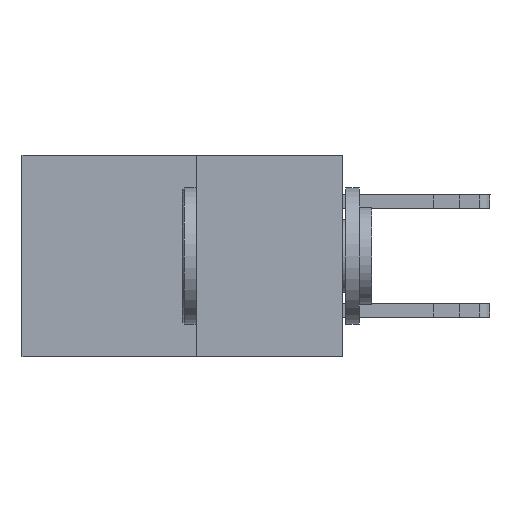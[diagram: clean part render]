
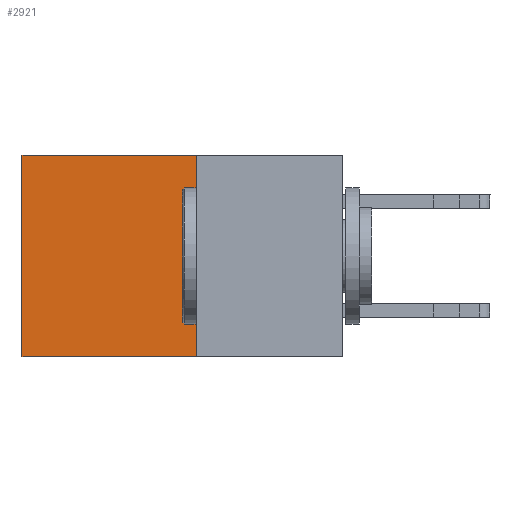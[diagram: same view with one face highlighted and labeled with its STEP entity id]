
A CAD part, left-side view. The second image highlights one B-rep face of the part: STEP entity #2921.
In plain terms, the highlighted planar face has unit normal (-1, 0, 0).
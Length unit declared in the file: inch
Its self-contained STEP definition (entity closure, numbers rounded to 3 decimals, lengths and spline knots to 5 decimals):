
#96 = LINE ( 'NONE', #9921, #3054 ) ;
#958 = VECTOR ( 'NONE', #9439, 39.37008 ) ;
#1492 = DIRECTION ( 'NONE',  ( 0., 0., -1. ) ) ;
#1629 = CARTESIAN_POINT ( 'NONE',  ( 0.277, 0.27, -0.37 ) ) ;
#1982 = DIRECTION ( 'NONE',  ( 0., 0., -1. ) ) ;
#2193 = VERTEX_POINT ( 'NONE', #3364 ) ;
#2755 = VECTOR ( 'NONE', #5610, 39.37008 ) ;
#2921 = ADVANCED_FACE ( 'NONE', ( #11876 ), #14265, .F. ) ;
#3054 = VECTOR ( 'NONE', #1492, 39.37008 ) ;
#3336 = AXIS2_PLACEMENT_3D ( 'NONE', #6869, #14428, #7793 ) ;
#3364 = CARTESIAN_POINT ( 'NONE',  ( 0.277, 0.27, 0. ) ) ;
#4204 = ORIENTED_EDGE ( 'NONE', *, *, #13382, .T. ) ;
#4409 = VECTOR ( 'NONE', #1982, 39.37008 ) ;
#5209 = ORIENTED_EDGE ( 'NONE', *, *, #8585, .F. ) ;
#5610 = DIRECTION ( 'NONE',  ( 0., 1., 0. ) ) ;
#5645 = EDGE_CURVE ( 'NONE', #5677, #10292, #15283, .T. ) ;
#5647 = CARTESIAN_POINT ( 'NONE',  ( 0.277, 0.59, -0.37 ) ) ;
#5677 = VERTEX_POINT ( 'NONE', #1629 ) ;
#6869 = CARTESIAN_POINT ( 'NONE',  ( 0.277, 0.27, -0.37 ) ) ;
#7793 = DIRECTION ( 'NONE',  ( 0., 0., -1. ) ) ;
#7897 = EDGE_LOOP ( 'NONE', ( #11575, #10295, #5209, #4204 ) ) ;
#8185 = CARTESIAN_POINT ( 'NONE',  ( 0.277, 0.59, 0. ) ) ;
#8585 = EDGE_CURVE ( 'NONE', #2193, #5677, #96, .T. ) ;
#9280 = LINE ( 'NONE', #13051, #958 ) ;
#9439 = DIRECTION ( 'NONE',  ( 0., 1., 0. ) ) ;
#9921 = CARTESIAN_POINT ( 'NONE',  ( 0.277, 0.27, -0.37 ) ) ;
#10292 = VERTEX_POINT ( 'NONE', #13553 ) ;
#10295 = ORIENTED_EDGE ( 'NONE', *, *, #5645, .F. ) ;
#10540 = CARTESIAN_POINT ( 'NONE',  ( 0.277, 0.27, -0.37 ) ) ;
#10567 = LINE ( 'NONE', #5647, #4409 ) ;
#11575 = ORIENTED_EDGE ( 'NONE', *, *, #15371, .T. ) ;
#11876 = FACE_OUTER_BOUND ( 'NONE', #7897, .T. ) ;
#13051 = CARTESIAN_POINT ( 'NONE',  ( 0.277, 0.27, 0. ) ) ;
#13382 = EDGE_CURVE ( 'NONE', #2193, #15328, #9280, .T. ) ;
#13553 = CARTESIAN_POINT ( 'NONE',  ( 0.277, 0.59, -0.37 ) ) ;
#14265 = PLANE ( 'NONE',  #3336 ) ;
#14428 = DIRECTION ( 'NONE',  ( 1., 0., 0. ) ) ;
#15283 = LINE ( 'NONE', #10540, #2755 ) ;
#15328 = VERTEX_POINT ( 'NONE', #8185 ) ;
#15371 = EDGE_CURVE ( 'NONE', #15328, #10292, #10567, .T. ) ;
